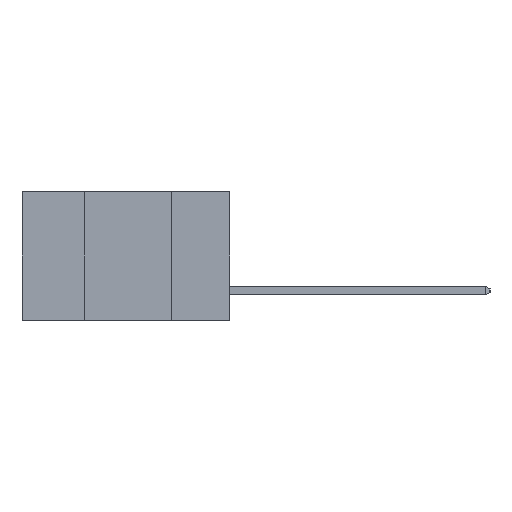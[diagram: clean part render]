
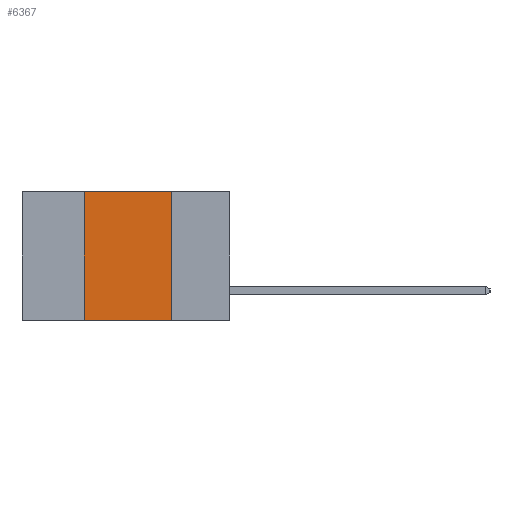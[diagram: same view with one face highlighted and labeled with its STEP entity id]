
A CAD part, left-side view. The second image highlights one B-rep face of the part: STEP entity #6367.
In plain terms, the highlighted planar face has unit normal (-1, 0, 0).
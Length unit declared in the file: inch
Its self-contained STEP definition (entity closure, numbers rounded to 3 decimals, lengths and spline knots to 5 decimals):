
#144 = CARTESIAN_POINT ( 'NONE',  ( 0., 0.17, -0.37 ) ) ;
#1387 = CARTESIAN_POINT ( 'NONE',  ( 0., 0.6, -0.37 ) ) ;
#1556 = DIRECTION ( 'NONE',  ( 0., -1., 0. ) ) ;
#2548 = LINE ( 'NONE', #12763, #10533 ) ;
#2620 = ORIENTED_EDGE ( 'NONE', *, *, #6660, .T. ) ;
#4213 = EDGE_LOOP ( 'NONE', ( #15975, #19064, #17158, #2620 ) ) ;
#4874 = DIRECTION ( 'NONE',  ( 0., 0., -1. ) ) ;
#5385 = VERTEX_POINT ( 'NONE', #14273 ) ;
#5739 = DIRECTION ( 'NONE',  ( 0., 0., 1. ) ) ;
#6367 = ADVANCED_FACE ( 'NONE', ( #20143 ), #8941, .F. ) ;
#6660 = EDGE_CURVE ( 'NONE', #5385, #14986, #15401, .T. ) ;
#6761 = DIRECTION ( 'NONE',  ( 0., -1., 0. ) ) ;
#8189 = DIRECTION ( 'NONE',  ( 0., 0., -1. ) ) ;
#8252 = DIRECTION ( 'NONE',  ( 1., 0., 0. ) ) ;
#8350 = CARTESIAN_POINT ( 'NONE',  ( 0., 0.6, 0. ) ) ;
#8941 = PLANE ( 'NONE',  #16197 ) ;
#10533 = VECTOR ( 'NONE', #4874, 39.37008 ) ;
#11323 = VECTOR ( 'NONE', #1556, 39.37008 ) ;
#12067 = CARTESIAN_POINT ( 'NONE',  ( 0., 0.42, -0.37 ) ) ;
#12479 = LINE ( 'NONE', #12067, #20093 ) ;
#12671 = VECTOR ( 'NONE', #6761, 39.37008 ) ;
#12763 = CARTESIAN_POINT ( 'NONE',  ( 0., 0.17, -0.37 ) ) ;
#13023 = VERTEX_POINT ( 'NONE', #18161 ) ;
#13035 = EDGE_CURVE ( 'NONE', #5385, #19193, #12479, .T. ) ;
#13058 = CARTESIAN_POINT ( 'NONE',  ( 0., 0.6, 0. ) ) ;
#13167 = LINE ( 'NONE', #13058, #12671 ) ;
#14273 = CARTESIAN_POINT ( 'NONE',  ( 0., 0.42, -0.37 ) ) ;
#14986 = VERTEX_POINT ( 'NONE', #144 ) ;
#15053 = EDGE_CURVE ( 'NONE', #19193, #13023, #13167, .T. ) ;
#15401 = LINE ( 'NONE', #1387, #11323 ) ;
#15975 = ORIENTED_EDGE ( 'NONE', *, *, #17140, .F. ) ;
#16197 = AXIS2_PLACEMENT_3D ( 'NONE', #8350, #8252, #8189 ) ;
#17140 = EDGE_CURVE ( 'NONE', #13023, #14986, #2548, .T. ) ;
#17158 = ORIENTED_EDGE ( 'NONE', *, *, #13035, .F. ) ;
#18161 = CARTESIAN_POINT ( 'NONE',  ( 0., 0.17, 0. ) ) ;
#18766 = CARTESIAN_POINT ( 'NONE',  ( 0., 0.42, 0. ) ) ;
#19064 = ORIENTED_EDGE ( 'NONE', *, *, #15053, .F. ) ;
#19193 = VERTEX_POINT ( 'NONE', #18766 ) ;
#20093 = VECTOR ( 'NONE', #5739, 39.37008 ) ;
#20143 = FACE_OUTER_BOUND ( 'NONE', #4213, .T. ) ;
